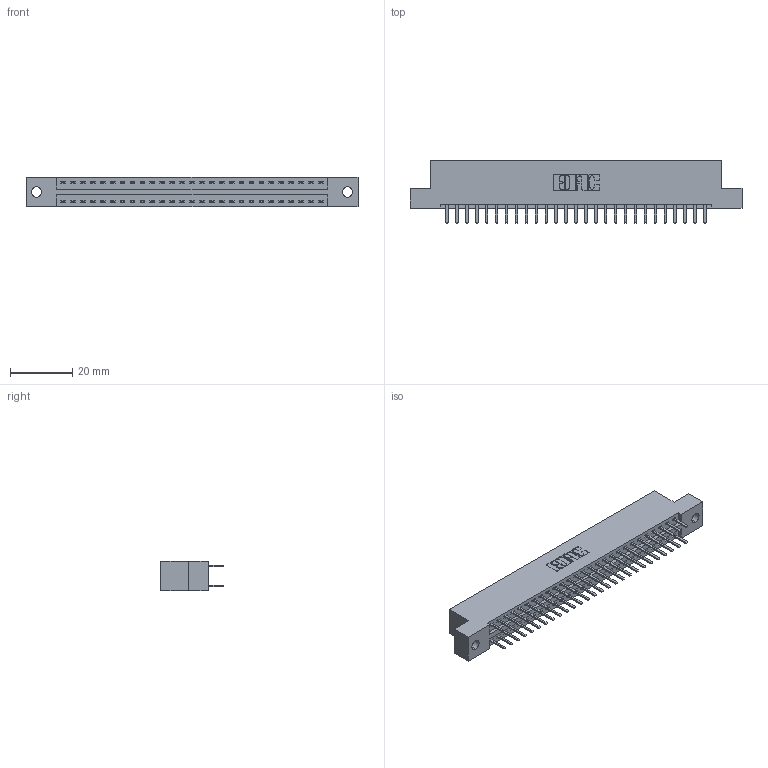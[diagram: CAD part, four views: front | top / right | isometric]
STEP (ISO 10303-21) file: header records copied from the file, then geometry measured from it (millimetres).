
FILE_DESCRIPTION (( 'STEP AP203' ), '1' );
FILE_NAME ('396-054-520-202.STEP', '2019-10-30T13:58:21', ( '' ), ( '' ), 'SwSTEP 2.0', 'SolidWorks 2016', '' );
FILE_SCHEMA (( 'CONFIG_CONTROL_DESIGN' ));
Length unit declared in the file: inch
Products named in the file (3): 396-054-520-202; 345-292-001_345-293-120; 346 Part_Flush Mounting Lugs - 0.128 Dia
Assembly tree (55 placements, depth 2):
  396-054-520-202
    346 Part_Flush Mounting Lugs - 0.128 Dia
    345-292-001_345-293-120  x54
Bounding box: 106.3 x 20.02 x 9.4 mm (x, y, z)
Volume: 10188.5 mm3; surface area: 13444.2 mm2
Topology: 55 solids, 55 shells, 3146 faces, 9131 edges, 5942 vertices
Faces by surface type: plane 2074, cylinder 1072
Entity records: 19757 total; most frequent: CARTESIAN_POINT 3288, ORIENTED_EDGE 3210, DIRECTION 2937, EDGE_CURVE 1605, VECTOR 1361, LINE 1361, VERTEX_POINT 1066, AXIS2_PLACEMENT_3D 788
